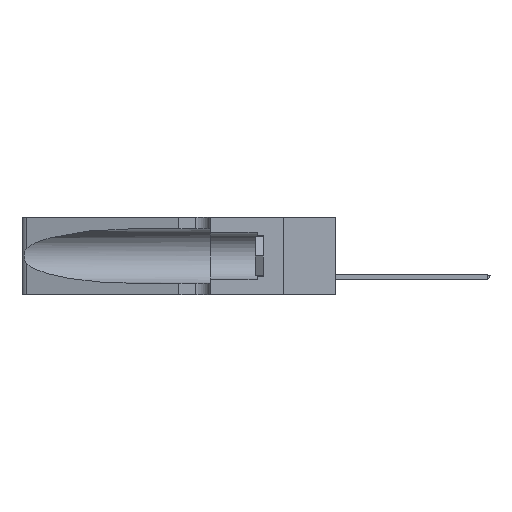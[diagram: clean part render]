
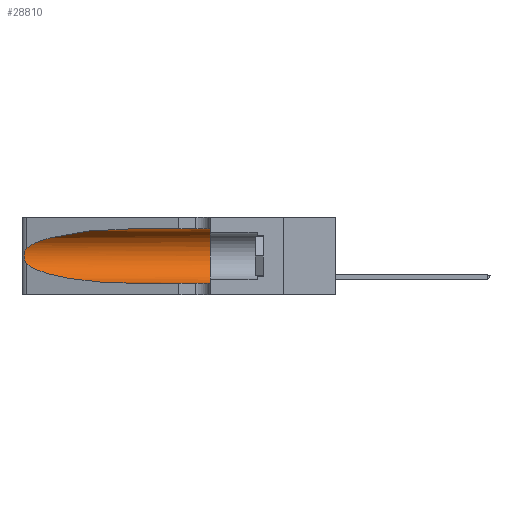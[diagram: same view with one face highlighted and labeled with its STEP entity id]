
A CAD part, left-side view. The second image highlights one B-rep face of the part: STEP entity #28810.
In plain terms, the highlighted cylindrical face has radius 3.308 mm (diameter 6.617 mm), a partial arc.
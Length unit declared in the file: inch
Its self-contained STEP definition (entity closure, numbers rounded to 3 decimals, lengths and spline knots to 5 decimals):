
#506 = ORIENTED_EDGE ( 'NONE', *, *, #27250, .F. ) ;
#871 = CARTESIAN_POINT ( 'NONE',  ( 0.26018, 1.23835, 0.19895 ) ) ;
#2962 = VECTOR ( 'NONE', #34662, 39.37008 ) ;
#3964 = CARTESIAN_POINT ( 'NONE',  ( 0.1305, 0.35, 0.185 ) ) ;
#4643 = CARTESIAN_POINT ( 'NONE',  ( 0.1305, 1.61858, 0.05475 ) ) ;
#5209 = CARTESIAN_POINT ( 'NONE',  ( 0.1305, 0.72297, 0.31525 ) ) ;
#6159 = CARTESIAN_POINT ( 'NONE',  ( 0.25487, 1.22718, 0.14631 ) ) ;
#6753 = CARTESIAN_POINT ( 'NONE',  ( 0.1305, 0.35, 0.05475 ) ) ;
#7055 = ORIENTED_EDGE ( 'NONE', *, *, #25528, .T. ) ;
#7083 = AXIS2_PLACEMENT_3D ( 'NONE', #3964, #37403, #37707 ) ;
#7474 = CARTESIAN_POINT ( 'NONE',  ( 0.26017, 1.23833, 0.17102 ) ) ;
#7790 = CARTESIAN_POINT ( 'NONE',  ( 0.18966, 0.96281, 0.05475 ) ) ;
#8021 = CARTESIAN_POINT ( 'NONE',  ( 0.25487, 1.22718, 0.22369 ) ) ;
#8688 = ORIENTED_EDGE ( 'NONE', *, *, #32174, .F. ) ;
#8937 = DIRECTION ( 'NONE',  ( 0., -1., 0. ) ) ;
#9759 = VECTOR ( 'NONE', #8937, 39.37008 ) ;
#10749 = CARTESIAN_POINT ( 'NONE',  ( 0.25789, 1.23486, 0.15765 ) ) ;
#10897 = CARTESIAN_POINT ( 'NONE',  ( 0.26075, 1.23896, 0.19203 ) ) ;
#11816 = EDGE_LOOP ( 'NONE', ( #33201, #22443, #18613, #7055, #506, #8688 ) ) ;
#14166 = CARTESIAN_POINT ( 'NONE',  ( 0.25854, 1.2359, 0.20912 ) ) ;
#14315 = CARTESIAN_POINT ( 'NONE',  ( 0.25856, 1.23593, 0.16098 ) ) ;
#14868 = CARTESIAN_POINT ( 'NONE',  ( 0.1305, 0.72297, 0.31525 ) ) ;
#16045 = DIRECTION ( 'NONE',  ( 0., -1., 0. ) ) ;
#16179 = LINE ( 'NONE', #43091, #9759 ) ;
#16320 = EDGE_CURVE ( 'NONE', #26771, #25203, #20971, .T. ) ;
#17882 = CARTESIAN_POINT ( 'NONE',  ( 0.25639, 1.23186, 0.15144 ) ) ;
#18024 = CARTESIAN_POINT ( 'NONE',  ( 0.25639, 1.23184, 0.21858 ) ) ;
#18263 = CARTESIAN_POINT ( 'NONE',  ( 0.18966, 0.96281, 0.31525 ) ) ;
#18613 = ORIENTED_EDGE ( 'NONE', *, *, #22116, .T. ) ;
#19077 =( BOUNDED_CURVE ( )  B_SPLINE_CURVE ( 3, ( #14868, #18263, #28654, #24962 ),
 .UNSPECIFIED., .F., .F. ) 
 B_SPLINE_CURVE_WITH_KNOTS ( ( 4, 4 ),
 ( 1.5708, 2.84003 ),
 .UNSPECIFIED. ) 
 CURVE ( )  GEOMETRIC_REPRESENTATION_ITEM ( )  RATIONAL_B_SPLINE_CURVE ( ( 1., 0.87, 0.87, 1. ) ) 
 REPRESENTATION_ITEM ( '' )  );
#20971 = B_SPLINE_CURVE_WITH_KNOTS ( 'NONE', 3,
 ( #38226, #24255, #18024, #24701, #14166, #871, #10897, #24841, #7474, #14315, #10749, #17882, #38075, #41758 ),
 .UNSPECIFIED., .F., .F.,
 ( 4, 2, 2, 2, 2, 2, 4 ),
 ( 0., 0.00027, 0.00053, 0.00107, 0.0016, 0.00187, 0.00214 ),
 .UNSPECIFIED. ) ;
#20987 =( BOUNDED_CURVE ( )  B_SPLINE_CURVE ( 3, ( #31414, #28560, #7790, #41635 ),
 .UNSPECIFIED., .F., .F. ) 
 B_SPLINE_CURVE_WITH_KNOTS ( ( 4, 4 ),
 ( 3.44316, 4.71239 ),
 .UNSPECIFIED. ) 
 CURVE ( )  GEOMETRIC_REPRESENTATION_ITEM ( )  RATIONAL_B_SPLINE_CURVE ( ( 1., 0.87, 0.87, 1. ) ) 
 REPRESENTATION_ITEM ( '' )  );
#22116 = EDGE_CURVE ( 'NONE', #25203, #37002, #20987, .T. ) ;
#22443 = ORIENTED_EDGE ( 'NONE', *, *, #16320, .T. ) ;
#24255 = CARTESIAN_POINT ( 'NONE',  ( 0.25555, 1.22994, 0.2215 ) ) ;
#24296 = EDGE_CURVE ( 'NONE', #30161, #26771, #19077, .T. ) ;
#24701 = CARTESIAN_POINT ( 'NONE',  ( 0.25787, 1.23484, 0.2124 ) ) ;
#24790 = AXIS2_PLACEMENT_3D ( 'NONE', #43066, #16045, #25658 ) ;
#24841 = CARTESIAN_POINT ( 'NONE',  ( 0.26075, 1.23896, 0.178 ) ) ;
#24962 = CARTESIAN_POINT ( 'NONE',  ( 0.25487, 1.22718, 0.22369 ) ) ;
#25160 = CARTESIAN_POINT ( 'NONE',  ( 0.1305, 0.72297, 0.05475 ) ) ;
#25203 = VERTEX_POINT ( 'NONE', #6159 ) ;
#25528 = EDGE_CURVE ( 'NONE', #37002, #41459, #41268, .T. ) ;
#25658 = DIRECTION ( 'NONE',  ( 0., 0., -1. ) ) ;
#26771 = VERTEX_POINT ( 'NONE', #8021 ) ;
#27250 = EDGE_CURVE ( 'NONE', #35661, #41459, #29413, .T. ) ;
#28560 = CARTESIAN_POINT ( 'NONE',  ( 0.2373, 1.15595, 0.08982 ) ) ;
#28654 = CARTESIAN_POINT ( 'NONE',  ( 0.2373, 1.15595, 0.28018 ) ) ;
#28810 = ADVANCED_FACE ( 'NONE', ( #32392 ), #31828, .F. ) ;
#29413 = CIRCLE ( 'NONE', #7083, 0.13025 ) ;
#30161 = VERTEX_POINT ( 'NONE', #5209 ) ;
#31414 = CARTESIAN_POINT ( 'NONE',  ( 0.25487, 1.22718, 0.14631 ) ) ;
#31828 = CYLINDRICAL_SURFACE ( 'NONE', #24790, 0.13025 ) ;
#32174 = EDGE_CURVE ( 'NONE', #30161, #35661, #16179, .T. ) ;
#32295 = CARTESIAN_POINT ( 'NONE',  ( 0.1305, 0.35, 0.31525 ) ) ;
#32392 = FACE_OUTER_BOUND ( 'NONE', #11816, .T. ) ;
#33201 = ORIENTED_EDGE ( 'NONE', *, *, #24296, .T. ) ;
#34662 = DIRECTION ( 'NONE',  ( 0., -1., 0. ) ) ;
#35661 = VERTEX_POINT ( 'NONE', #32295 ) ;
#37002 = VERTEX_POINT ( 'NONE', #25160 ) ;
#37403 = DIRECTION ( 'NONE',  ( 0., 1., 0. ) ) ;
#37707 = DIRECTION ( 'NONE',  ( 0., 0., 1. ) ) ;
#38075 = CARTESIAN_POINT ( 'NONE',  ( 0.25555, 1.22993, 0.14849 ) ) ;
#38226 = CARTESIAN_POINT ( 'NONE',  ( 0.25487, 1.22718, 0.22369 ) ) ;
#41268 = LINE ( 'NONE', #4643, #2962 ) ;
#41459 = VERTEX_POINT ( 'NONE', #6753 ) ;
#41635 = CARTESIAN_POINT ( 'NONE',  ( 0.1305, 0.72297, 0.05475 ) ) ;
#41758 = CARTESIAN_POINT ( 'NONE',  ( 0.25487, 1.22718, 0.14631 ) ) ;
#43066 = CARTESIAN_POINT ( 'NONE',  ( 0.1305, 1.61858, 0.185 ) ) ;
#43091 = CARTESIAN_POINT ( 'NONE',  ( 0.1305, 1.61858, 0.31525 ) ) ;
